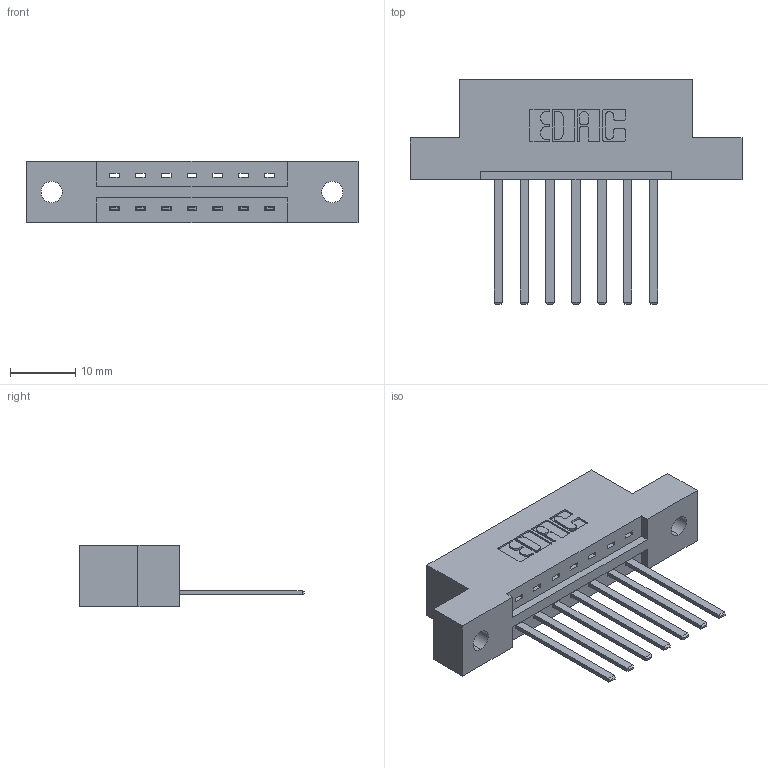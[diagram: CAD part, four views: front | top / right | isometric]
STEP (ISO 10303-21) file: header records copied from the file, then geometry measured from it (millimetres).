
FILE_DESCRIPTION (( 'STEP AP203' ), '1' );
FILE_NAME ('387-007-544-102.STEP', '2019-10-02T02:39:20', ( '' ), ( '' ), 'SwSTEP 2.0', 'SolidWorks 2016', '' );
FILE_SCHEMA (( 'CONFIG_CONTROL_DESIGN' ));
Length unit declared in the file: inch
Products named in the file (3): 345-292-001_345-293-144; 337 Part_Flush Mounting Lugs - 0.128 Dia; 387-007-544-102
Assembly tree (8 placements, depth 2):
  387-007-544-102
    337 Part_Flush Mounting Lugs - 0.128 Dia
    345-292-001_345-293-144  x7
Bounding box: 50.75 x 34.3 x 9.4 mm (x, y, z)
Volume: 4880.9 mm3; surface area: 4846.3 mm2
Topology: 8 solids, 8 shells, 506 faces, 1501 edges, 990 vertices
Faces by surface type: plane 364, cylinder 142
Entity records: 9549 total; most frequent: CARTESIAN_POINT 1667, ORIENTED_EDGE 1610, DIRECTION 1471, EDGE_CURVE 805, LINE 681, VECTOR 681, VERTEX_POINT 534, AXIS2_PLACEMENT_3D 395
